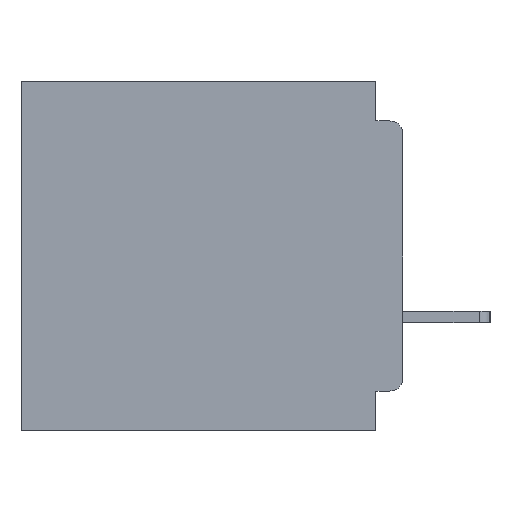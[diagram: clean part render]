
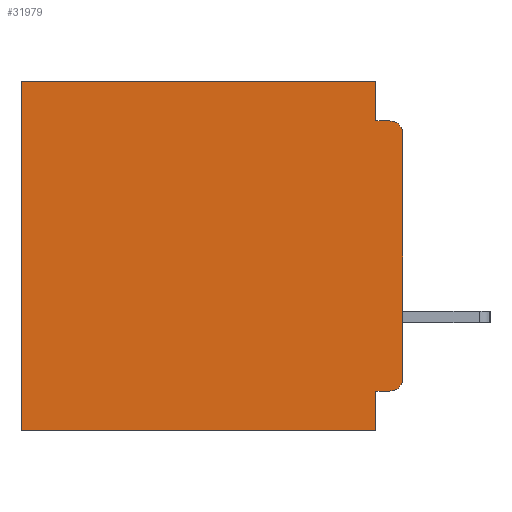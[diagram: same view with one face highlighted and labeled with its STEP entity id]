
A CAD part, left-side view. The second image highlights one B-rep face of the part: STEP entity #31979.
In plain terms, the highlighted planar face has unit normal (-1, 0, 0).
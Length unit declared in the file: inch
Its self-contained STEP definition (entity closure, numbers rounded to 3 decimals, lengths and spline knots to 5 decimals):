
#629 = DIRECTION ( 'NONE',  ( 0., 0., -1. ) ) ;
#875 = CARTESIAN_POINT ( 'NONE',  ( 0.3, 0.031, -0.355 ) ) ;
#2147 = CARTESIAN_POINT ( 'NONE',  ( 0.3, 0.015, -0.34 ) ) ;
#2986 = AXIS2_PLACEMENT_3D ( 'NONE', #6334, #37594, #10944 ) ;
#3260 = VERTEX_POINT ( 'NONE', #40608 ) ;
#4055 = EDGE_CURVE ( 'NONE', #38525, #10185, #34135, .T. ) ;
#4146 = DIRECTION ( 'NONE',  ( 0., 0., -1. ) ) ;
#4173 = DIRECTION ( 'NONE',  ( 0., 0., -1. ) ) ;
#4413 = EDGE_CURVE ( 'NONE', #52882, #16322, #40973, .T. ) ;
#4523 = CARTESIAN_POINT ( 'NONE',  ( 0.3, 0.437, -0.4 ) ) ;
#4777 = ORIENTED_EDGE ( 'NONE', *, *, #12459, .F. ) ;
#4985 = CARTESIAN_POINT ( 'NONE',  ( 0.3, 0.437, -0.4 ) ) ;
#5320 = VECTOR ( 'NONE', #33384, 39.37008 ) ;
#5463 = VECTOR ( 'NONE', #55452, 39.37008 ) ;
#5694 = FACE_OUTER_BOUND ( 'NONE', #34460, .T. ) ;
#6156 = VECTOR ( 'NONE', #4146, 39.37008 ) ;
#6334 = CARTESIAN_POINT ( 'NONE',  ( 0.3, 0.015, -0.06 ) ) ;
#6739 = DIRECTION ( 'NONE',  ( 0., 0., -1. ) ) ;
#6797 = VERTEX_POINT ( 'NONE', #42390 ) ;
#7109 = EDGE_CURVE ( 'NONE', #3260, #32907, #57579, .T. ) ;
#7916 = EDGE_CURVE ( 'NONE', #16322, #47744, #35633, .T. ) ;
#10185 = VERTEX_POINT ( 'NONE', #45771 ) ;
#10944 = DIRECTION ( 'NONE',  ( 0., 0., -1. ) ) ;
#12459 = EDGE_CURVE ( 'NONE', #52882, #14397, #41796, .T. ) ;
#14397 = VERTEX_POINT ( 'NONE', #18074 ) ;
#16322 = VERTEX_POINT ( 'NONE', #32669 ) ;
#18074 = CARTESIAN_POINT ( 'NONE',  ( 0.3, 0.031, -0.045 ) ) ;
#18557 = VERTEX_POINT ( 'NONE', #42415 ) ;
#19563 = CIRCLE ( 'NONE', #42184, 0.015 ) ;
#19927 = DIRECTION ( 'NONE',  ( 0., 1., 0. ) ) ;
#20629 = CARTESIAN_POINT ( 'NONE',  ( 0.3, 0., -0.355 ) ) ;
#21675 = CARTESIAN_POINT ( 'NONE',  ( 0.3, 0., -0.4 ) ) ;
#22117 = CARTESIAN_POINT ( 'NONE',  ( 0.3, 0.031, 0. ) ) ;
#23815 = LINE ( 'NONE', #37550, #43183 ) ;
#23865 = VECTOR ( 'NONE', #4173, 39.37008 ) ;
#25617 = EDGE_CURVE ( 'NONE', #6797, #38525, #47338, .T. ) ;
#25809 = AXIS2_PLACEMENT_3D ( 'NONE', #21675, #47964, #56818 ) ;
#26176 = EDGE_CURVE ( 'NONE', #6797, #32907, #19563, .T. ) ;
#26679 = CIRCLE ( 'NONE', #2986, 0.015 ) ;
#29215 = CARTESIAN_POINT ( 'NONE',  ( 0.3, 0., -0.045 ) ) ;
#29556 = ORIENTED_EDGE ( 'NONE', *, *, #4055, .F. ) ;
#31577 = ORIENTED_EDGE ( 'NONE', *, *, #25617, .F. ) ;
#31954 = ORIENTED_EDGE ( 'NONE', *, *, #26176, .T. ) ;
#31979 = ADVANCED_FACE ( 'NONE', ( #5694 ), #48152, .F. ) ;
#32669 = CARTESIAN_POINT ( 'NONE',  ( 0.3, 0.437, 0. ) ) ;
#32907 = VERTEX_POINT ( 'NONE', #41529 ) ;
#33384 = DIRECTION ( 'NONE',  ( 0., 1., 0. ) ) ;
#33578 = DIRECTION ( 'NONE',  ( -1., 0., 0. ) ) ;
#34135 = LINE ( 'NONE', #41794, #55978 ) ;
#34460 = EDGE_LOOP ( 'NONE', ( #46396, #41828, #35480, #4777, #56495, #42355, #42314, #29556, #31577, #31954 ) ) ;
#35480 = ORIENTED_EDGE ( 'NONE', *, *, #40043, .F. ) ;
#35633 = LINE ( 'NONE', #4523, #23865 ) ;
#37550 = CARTESIAN_POINT ( 'NONE',  ( 0.3, 0., -0.4 ) ) ;
#37594 = DIRECTION ( 'NONE',  ( -1., 0., 0. ) ) ;
#37721 = CARTESIAN_POINT ( 'NONE',  ( 0.3, 0., 0. ) ) ;
#38263 = DIRECTION ( 'NONE',  ( 0., 1., 0. ) ) ;
#38525 = VERTEX_POINT ( 'NONE', #875 ) ;
#40043 = EDGE_CURVE ( 'NONE', #14397, #18557, #52721, .T. ) ;
#40608 = CARTESIAN_POINT ( 'NONE',  ( 0.3, 0., -0.06 ) ) ;
#40973 = LINE ( 'NONE', #37721, #5320 ) ;
#41529 = CARTESIAN_POINT ( 'NONE',  ( 0.3, 0., -0.34 ) ) ;
#41794 = CARTESIAN_POINT ( 'NONE',  ( 0.3, 0.031, -0.4 ) ) ;
#41796 = LINE ( 'NONE', #22117, #6156 ) ;
#41828 = ORIENTED_EDGE ( 'NONE', *, *, #54582, .T. ) ;
#42184 = AXIS2_PLACEMENT_3D ( 'NONE', #2147, #33578, #6739 ) ;
#42314 = ORIENTED_EDGE ( 'NONE', *, *, #55086, .F. ) ;
#42355 = ORIENTED_EDGE ( 'NONE', *, *, #7916, .T. ) ;
#42390 = CARTESIAN_POINT ( 'NONE',  ( 0.3, 0.015, -0.355 ) ) ;
#42415 = CARTESIAN_POINT ( 'NONE',  ( 0.3, 0.015, -0.045 ) ) ;
#43183 = VECTOR ( 'NONE', #19927, 39.37008 ) ;
#44724 = VECTOR ( 'NONE', #53148, 39.37008 ) ;
#45771 = CARTESIAN_POINT ( 'NONE',  ( 0.3, 0.031, -0.4 ) ) ;
#46396 = ORIENTED_EDGE ( 'NONE', *, *, #7109, .F. ) ;
#47338 = LINE ( 'NONE', #20629, #48660 ) ;
#47744 = VERTEX_POINT ( 'NONE', #4985 ) ;
#47964 = DIRECTION ( 'NONE',  ( 1., 0., 0. ) ) ;
#48152 = PLANE ( 'NONE',  #25809 ) ;
#48660 = VECTOR ( 'NONE', #38263, 39.37008 ) ;
#52716 = CARTESIAN_POINT ( 'NONE',  ( 0.3, 0., -0.4 ) ) ;
#52721 = LINE ( 'NONE', #29215, #5463 ) ;
#52882 = VERTEX_POINT ( 'NONE', #56925 ) ;
#53148 = DIRECTION ( 'NONE',  ( 0., 0., -1. ) ) ;
#54582 = EDGE_CURVE ( 'NONE', #3260, #18557, #26679, .T. ) ;
#55086 = EDGE_CURVE ( 'NONE', #10185, #47744, #23815, .T. ) ;
#55452 = DIRECTION ( 'NONE',  ( 0., -1., 0. ) ) ;
#55978 = VECTOR ( 'NONE', #629, 39.37008 ) ;
#56495 = ORIENTED_EDGE ( 'NONE', *, *, #4413, .T. ) ;
#56818 = DIRECTION ( 'NONE',  ( 0., 0., -1. ) ) ;
#56925 = CARTESIAN_POINT ( 'NONE',  ( 0.3, 0.031, 0. ) ) ;
#57579 = LINE ( 'NONE', #52716, #44724 ) ;
